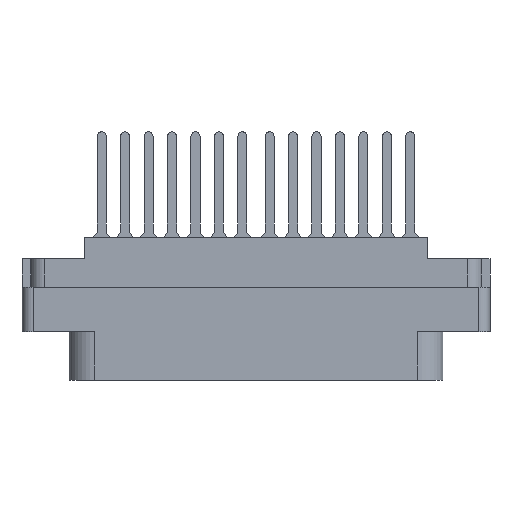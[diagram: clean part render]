
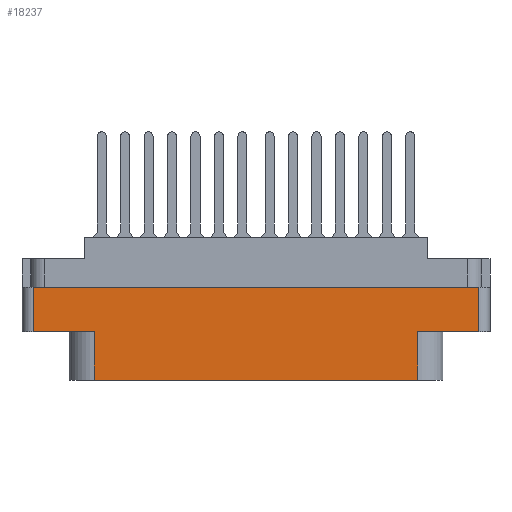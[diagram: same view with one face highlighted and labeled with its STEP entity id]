
A CAD part, front view. The second image highlights one B-rep face of the part: STEP entity #18237.
In plain terms, the highlighted planar face has unit normal (0, -1, 0).
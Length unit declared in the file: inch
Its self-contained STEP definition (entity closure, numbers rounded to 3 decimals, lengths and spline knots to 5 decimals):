
#33 = DIRECTION ( 'NONE',  ( 1., 0., 0. ) ) ;
#498 = DIRECTION ( 'NONE',  ( -1., 0., 0. ) ) ;
#3083 = EDGE_CURVE ( 'NONE', #16675, #40750, #44177, .T. ) ;
#3745 = DIRECTION ( 'NONE',  ( 0., 0., 1. ) ) ;
#3763 = DIRECTION ( 'NONE',  ( 0., 0., -1. ) ) ;
#4029 = ORIENTED_EDGE ( 'NONE', *, *, #4129, .T. ) ;
#4129 = EDGE_CURVE ( 'NONE', #23490, #41287, #44762, .T. ) ;
#4364 = LINE ( 'NONE', #21252, #18625 ) ;
#4373 = AXIS2_PLACEMENT_3D ( 'NONE', #8605, #8335, #7916 ) ;
#4759 = EDGE_CURVE ( 'NONE', #23490, #31747, #31852, .T. ) ;
#5296 = FACE_OUTER_BOUND ( 'NONE', #9527, .T. ) ;
#5929 = ORIENTED_EDGE ( 'NONE', *, *, #3083, .T. ) ;
#6493 = EDGE_CURVE ( 'NONE', #24475, #41287, #44879, .T. ) ;
#7543 = VECTOR ( 'NONE', #33, 39.37008 ) ;
#7916 = DIRECTION ( 'NONE',  ( 0., 0., -1. ) ) ;
#7986 = PLANE ( 'NONE',  #4373 ) ;
#8335 = DIRECTION ( 'NONE',  ( 0., -1., 0. ) ) ;
#8406 = VERTEX_POINT ( 'NONE', #27006 ) ;
#8605 = CARTESIAN_POINT ( 'NONE',  ( -1.2955, -0.438, -0.789 ) ) ;
#8839 = VECTOR ( 'NONE', #498, 39.37008 ) ;
#9488 = CARTESIAN_POINT ( 'NONE',  ( -0.895, -0.438, -0.52 ) ) ;
#9527 = EDGE_LOOP ( 'NONE', ( #31654, #22808, #28160, #27962, #5929, #14229, #11695, #4029 ) ) ;
#10154 = CARTESIAN_POINT ( 'NONE',  ( 1.2335, -0.438, -0.52 ) ) ;
#10635 = CARTESIAN_POINT ( 'NONE',  ( -0.895, -0.438, -0.789 ) ) ;
#10777 = EDGE_CURVE ( 'NONE', #24475, #8406, #4364, .T. ) ;
#11695 = ORIENTED_EDGE ( 'NONE', *, *, #4759, .F. ) ;
#13295 = CARTESIAN_POINT ( 'NONE',  ( 0.895, -0.438, -0.52 ) ) ;
#13830 = EDGE_CURVE ( 'NONE', #27766, #16675, #16773, .T. ) ;
#14229 = ORIENTED_EDGE ( 'NONE', *, *, #41387, .T. ) ;
#14551 = CARTESIAN_POINT ( 'NONE',  ( 0., -0.438, -0.52 ) ) ;
#16169 = CARTESIAN_POINT ( 'NONE',  ( -1.2955, -0.438, -0.789 ) ) ;
#16309 = CARTESIAN_POINT ( 'NONE',  ( 0.895, -0.438, -0.52 ) ) ;
#16675 = VERTEX_POINT ( 'NONE', #26184 ) ;
#16773 = LINE ( 'NONE', #10635, #30494 ) ;
#17562 = LINE ( 'NONE', #13295, #27436 ) ;
#18237 = ADVANCED_FACE ( 'NONE', ( #5296 ), #7986, .T. ) ;
#18625 = VECTOR ( 'NONE', #3763, 39.37008 ) ;
#20255 = DIRECTION ( 'NONE',  ( 0., 0., -1. ) ) ;
#20331 = DIRECTION ( 'NONE',  ( 0., 0., 1. ) ) ;
#21252 = CARTESIAN_POINT ( 'NONE',  ( -1.2335, -0.438, -0.789 ) ) ;
#22808 = ORIENTED_EDGE ( 'NONE', *, *, #10777, .T. ) ;
#23490 = VERTEX_POINT ( 'NONE', #10154 ) ;
#24475 = VERTEX_POINT ( 'NONE', #41616 ) ;
#26128 = CARTESIAN_POINT ( 'NONE',  ( 0., -0.438, -0.52 ) ) ;
#26184 = CARTESIAN_POINT ( 'NONE',  ( -0.895, -0.438, -0.789 ) ) ;
#27006 = CARTESIAN_POINT ( 'NONE',  ( -1.2335, -0.438, -0.52 ) ) ;
#27436 = VECTOR ( 'NONE', #20331, 39.37008 ) ;
#27766 = VERTEX_POINT ( 'NONE', #9488 ) ;
#27962 = ORIENTED_EDGE ( 'NONE', *, *, #13830, .T. ) ;
#28160 = ORIENTED_EDGE ( 'NONE', *, *, #37739, .F. ) ;
#29829 = DIRECTION ( 'NONE',  ( 1., 0., 0. ) ) ;
#30494 = VECTOR ( 'NONE', #20255, 39.37008 ) ;
#31654 = ORIENTED_EDGE ( 'NONE', *, *, #6493, .F. ) ;
#31747 = VERTEX_POINT ( 'NONE', #16309 ) ;
#31852 = LINE ( 'NONE', #26128, #8839 ) ;
#32039 = VECTOR ( 'NONE', #39103, 39.37008 ) ;
#33684 = CARTESIAN_POINT ( 'NONE',  ( 1.2335, -0.438, -0.274 ) ) ;
#37574 = VECTOR ( 'NONE', #29829, 39.37008 ) ;
#37739 = EDGE_CURVE ( 'NONE', #27766, #8406, #39752, .T. ) ;
#39103 = DIRECTION ( 'NONE',  ( -1., 0., 0. ) ) ;
#39443 = CARTESIAN_POINT ( 'NONE',  ( 0.895, -0.438, -0.789 ) ) ;
#39752 = LINE ( 'NONE', #14551, #32039 ) ;
#40750 = VERTEX_POINT ( 'NONE', #39443 ) ;
#41287 = VERTEX_POINT ( 'NONE', #33684 ) ;
#41387 = EDGE_CURVE ( 'NONE', #40750, #31747, #17562, .T. ) ;
#41616 = CARTESIAN_POINT ( 'NONE',  ( -1.2335, -0.438, -0.274 ) ) ;
#41913 = CARTESIAN_POINT ( 'NONE',  ( 0., -0.438, -0.274 ) ) ;
#42517 = VECTOR ( 'NONE', #3745, 39.37008 ) ;
#42701 = CARTESIAN_POINT ( 'NONE',  ( 1.2335, -0.438, -0.789 ) ) ;
#44177 = LINE ( 'NONE', #16169, #37574 ) ;
#44762 = LINE ( 'NONE', #42701, #42517 ) ;
#44879 = LINE ( 'NONE', #41913, #7543 ) ;
